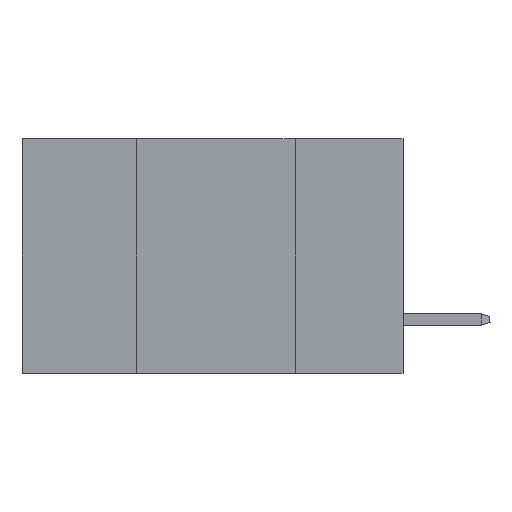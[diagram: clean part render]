
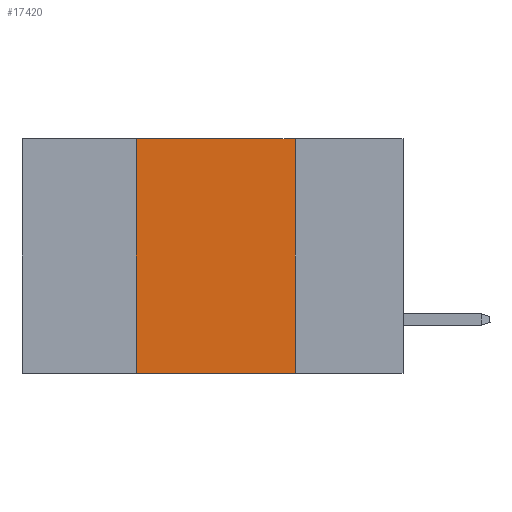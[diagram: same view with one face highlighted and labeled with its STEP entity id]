
A CAD part, left-side view. The second image highlights one B-rep face of the part: STEP entity #17420.
In plain terms, the highlighted planar face has unit normal (-1, 0, 0).
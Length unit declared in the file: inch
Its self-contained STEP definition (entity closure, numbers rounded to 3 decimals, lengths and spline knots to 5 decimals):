
#190 = EDGE_CURVE ( 'NONE', #15826, #18643, #21124, .T. ) ;
#1488 = FACE_OUTER_BOUND ( 'NONE', #2890, .T. ) ;
#1703 = EDGE_CURVE ( 'NONE', #8323, #15826, #17264, .T. ) ;
#2890 = EDGE_LOOP ( 'NONE', ( #12918, #23723, #3915, #12350 ) ) ;
#3915 = ORIENTED_EDGE ( 'NONE', *, *, #1703, .F. ) ;
#4777 = CARTESIAN_POINT ( 'NONE',  ( 0., 0.17, 0. ) ) ;
#6800 = VECTOR ( 'NONE', #18935, 39.37008 ) ;
#8323 = VERTEX_POINT ( 'NONE', #23049 ) ;
#9621 = EDGE_CURVE ( 'NONE', #18643, #20931, #15833, .T. ) ;
#9682 = CARTESIAN_POINT ( 'NONE',  ( 0., 0.42, 0. ) ) ;
#10886 = DIRECTION ( 'NONE',  ( 0., -1., 0. ) ) ;
#11176 = VECTOR ( 'NONE', #10886, 39.37008 ) ;
#12094 = DIRECTION ( 'NONE',  ( 0., 0., -1. ) ) ;
#12350 = ORIENTED_EDGE ( 'NONE', *, *, #15160, .T. ) ;
#12493 = VECTOR ( 'NONE', #19313, 39.37008 ) ;
#12918 = ORIENTED_EDGE ( 'NONE', *, *, #9621, .F. ) ;
#14129 = PLANE ( 'NONE',  #17401 ) ;
#14731 = CARTESIAN_POINT ( 'NONE',  ( 0., 0.6, -0.37 ) ) ;
#14844 = VECTOR ( 'NONE', #12094, 39.37008 ) ;
#15160 = EDGE_CURVE ( 'NONE', #8323, #20931, #16301, .T. ) ;
#15826 = VERTEX_POINT ( 'NONE', #23004 ) ;
#15833 = LINE ( 'NONE', #4777, #14844 ) ;
#16301 = LINE ( 'NONE', #14731, #11176 ) ;
#17264 = LINE ( 'NONE', #9682, #6800 ) ;
#17401 = AXIS2_PLACEMENT_3D ( 'NONE', #17829, #19649, #23383 ) ;
#17420 = ADVANCED_FACE ( 'NONE', ( #1488 ), #14129, .F. ) ;
#17829 = CARTESIAN_POINT ( 'NONE',  ( 0., 0.6, 0. ) ) ;
#17874 = CARTESIAN_POINT ( 'NONE',  ( 0., 0.6, 0. ) ) ;
#18643 = VERTEX_POINT ( 'NONE', #22606 ) ;
#18935 = DIRECTION ( 'NONE',  ( 0., 0., 1. ) ) ;
#18971 = CARTESIAN_POINT ( 'NONE',  ( 0., 0.17, -0.37 ) ) ;
#19313 = DIRECTION ( 'NONE',  ( 0., -1., 0. ) ) ;
#19649 = DIRECTION ( 'NONE',  ( 1., 0., 0. ) ) ;
#20931 = VERTEX_POINT ( 'NONE', #18971 ) ;
#21124 = LINE ( 'NONE', #17874, #12493 ) ;
#22606 = CARTESIAN_POINT ( 'NONE',  ( 0., 0.17, 0. ) ) ;
#23004 = CARTESIAN_POINT ( 'NONE',  ( 0., 0.42, 0. ) ) ;
#23049 = CARTESIAN_POINT ( 'NONE',  ( 0., 0.42, -0.37 ) ) ;
#23383 = DIRECTION ( 'NONE',  ( 0., 0., -1. ) ) ;
#23723 = ORIENTED_EDGE ( 'NONE', *, *, #190, .F. ) ;
